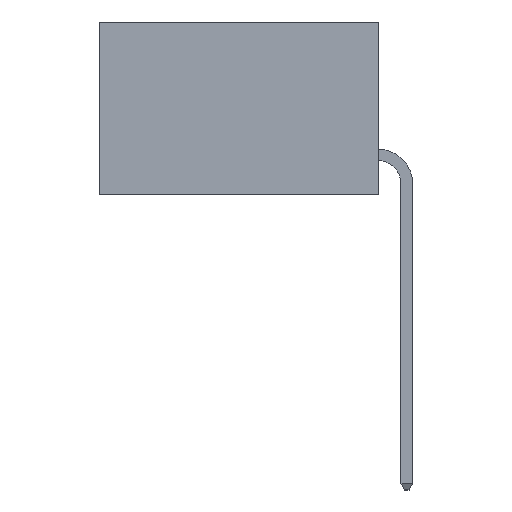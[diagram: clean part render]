
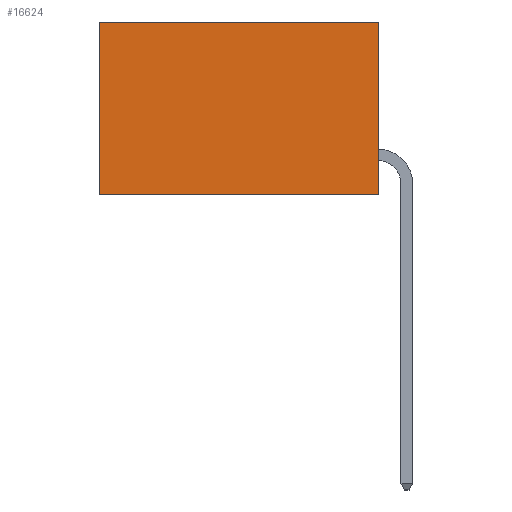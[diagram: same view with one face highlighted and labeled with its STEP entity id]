
A CAD part, left-side view. The second image highlights one B-rep face of the part: STEP entity #16624.
In plain terms, the highlighted planar face has unit normal (-1, 0, 0).
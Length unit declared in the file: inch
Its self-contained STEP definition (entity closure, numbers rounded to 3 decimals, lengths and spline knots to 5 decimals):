
#195 = EDGE_CURVE ( 'NONE', #3666, #15335, #13741, .T. ) ;
#207 = ORIENTED_EDGE ( 'NONE', *, *, #14545, .T. ) ;
#711 = CARTESIAN_POINT ( 'NONE',  ( 0.2615, 0.6, -0.37 ) ) ;
#1211 = LINE ( 'NONE', #1515, #4397 ) ;
#1515 = CARTESIAN_POINT ( 'NONE',  ( 0.2615, 0., 0. ) ) ;
#1612 = DIRECTION ( 'NONE',  ( 0., 0., -1. ) ) ;
#1855 = CARTESIAN_POINT ( 'NONE',  ( 0.2615, 0.6, -0.37 ) ) ;
#2678 = FACE_OUTER_BOUND ( 'NONE', #7852, .T. ) ;
#3666 = VERTEX_POINT ( 'NONE', #8357 ) ;
#3804 = EDGE_CURVE ( 'NONE', #7964, #4370, #12163, .T. ) ;
#4370 = VERTEX_POINT ( 'NONE', #7232 ) ;
#4397 = VECTOR ( 'NONE', #9588, 39.37008 ) ;
#6420 = CARTESIAN_POINT ( 'NONE',  ( 0.2615, 0., -0.37 ) ) ;
#6459 = AXIS2_PLACEMENT_3D ( 'NONE', #7486, #16714, #8828 ) ;
#6574 = DIRECTION ( 'NONE',  ( 0., 0., -1. ) ) ;
#6873 = ORIENTED_EDGE ( 'NONE', *, *, #8541, .F. ) ;
#7011 = VECTOR ( 'NONE', #10435, 39.37008 ) ;
#7232 = CARTESIAN_POINT ( 'NONE',  ( 0.2615, 0., -0.37 ) ) ;
#7486 = CARTESIAN_POINT ( 'NONE',  ( 0.2615, 0., -0.37 ) ) ;
#7595 = ORIENTED_EDGE ( 'NONE', *, *, #195, .T. ) ;
#7852 = EDGE_LOOP ( 'NONE', ( #7595, #6873, #13830, #207 ) ) ;
#7964 = VERTEX_POINT ( 'NONE', #16178 ) ;
#8357 = CARTESIAN_POINT ( 'NONE',  ( 0.2615, 0.6, 0. ) ) ;
#8541 = EDGE_CURVE ( 'NONE', #4370, #15335, #10552, .T. ) ;
#8828 = DIRECTION ( 'NONE',  ( 0., 0., -1. ) ) ;
#9588 = DIRECTION ( 'NONE',  ( 0., 1., 0. ) ) ;
#10435 = DIRECTION ( 'NONE',  ( 0., 1., 0. ) ) ;
#10552 = LINE ( 'NONE', #10705, #7011 ) ;
#10705 = CARTESIAN_POINT ( 'NONE',  ( 0.2615, 0., -0.37 ) ) ;
#12163 = LINE ( 'NONE', #6420, #14870 ) ;
#13331 = VECTOR ( 'NONE', #1612, 39.37008 ) ;
#13741 = LINE ( 'NONE', #711, #13331 ) ;
#13830 = ORIENTED_EDGE ( 'NONE', *, *, #3804, .F. ) ;
#14545 = EDGE_CURVE ( 'NONE', #7964, #3666, #1211, .T. ) ;
#14870 = VECTOR ( 'NONE', #6574, 39.37008 ) ;
#15335 = VERTEX_POINT ( 'NONE', #1855 ) ;
#15428 = PLANE ( 'NONE',  #6459 ) ;
#16178 = CARTESIAN_POINT ( 'NONE',  ( 0.2615, 0., 0. ) ) ;
#16624 = ADVANCED_FACE ( 'NONE', ( #2678 ), #15428, .F. ) ;
#16714 = DIRECTION ( 'NONE',  ( 1., 0., 0. ) ) ;
